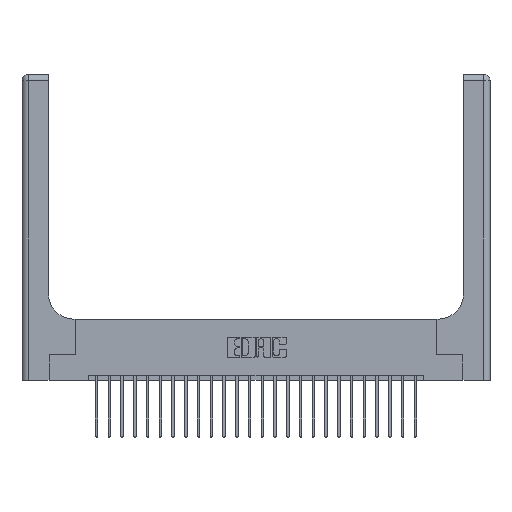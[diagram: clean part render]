
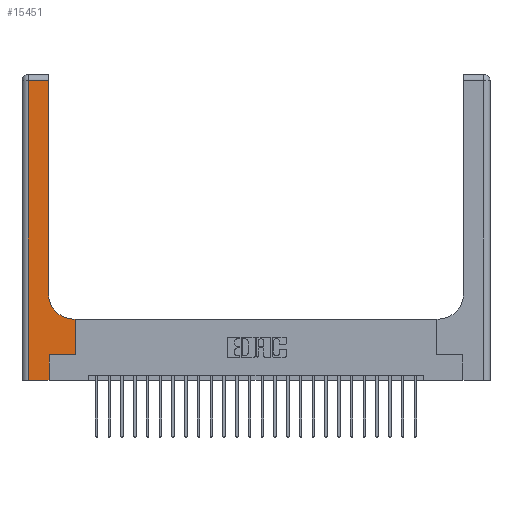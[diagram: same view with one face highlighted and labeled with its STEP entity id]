
A CAD part, top view. The second image highlights one B-rep face of the part: STEP entity #15451.
In plain terms, the highlighted planar face has unit normal (0, 0, 1).
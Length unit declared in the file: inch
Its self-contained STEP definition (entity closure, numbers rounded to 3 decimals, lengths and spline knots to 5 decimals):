
#1 = LINE ( 'NONE', #17012, #22369 ) ;
#165 = CARTESIAN_POINT ( 'NONE',  ( 0.26, 2.94, 0.37 ) ) ;
#623 = CARTESIAN_POINT ( 'NONE',  ( 0.06, 0., 0.37 ) ) ;
#660 = VECTOR ( 'NONE', #21914, 39.37008 ) ;
#692 = ORIENTED_EDGE ( 'NONE', *, *, #14863, .T. ) ;
#721 = DIRECTION ( 'NONE',  ( 0., 1., 0. ) ) ;
#759 = VECTOR ( 'NONE', #11160, 39.37008 ) ;
#1568 = DIRECTION ( 'NONE',  ( 0., 0., -1. ) ) ;
#1949 = DIRECTION ( 'NONE',  ( -1., 0., 0. ) ) ;
#2361 = DIRECTION ( 'NONE',  ( 0., 1., 0. ) ) ;
#2493 = VERTEX_POINT ( 'NONE', #22135 ) ;
#2516 = LINE ( 'NONE', #21000, #11321 ) ;
#2921 = EDGE_LOOP ( 'NONE', ( #4678, #18273, #2970, #3526, #19930, #16629, #23258, #692, #19348 ) ) ;
#2970 = ORIENTED_EDGE ( 'NONE', *, *, #20017, .T. ) ;
#2985 = EDGE_CURVE ( 'NONE', #14610, #8195, #4981, .T. ) ;
#3526 = ORIENTED_EDGE ( 'NONE', *, *, #21913, .T. ) ;
#4008 = DIRECTION ( 'NONE',  ( 0., -1., 0. ) ) ;
#4084 = CARTESIAN_POINT ( 'NONE',  ( 0.06, 3., 0.37 ) ) ;
#4603 = LINE ( 'NONE', #13674, #11667 ) ;
#4678 = ORIENTED_EDGE ( 'NONE', *, *, #7234, .T. ) ;
#4731 = VERTEX_POINT ( 'NONE', #165 ) ;
#4958 = VERTEX_POINT ( 'NONE', #623 ) ;
#4981 = LINE ( 'NONE', #6660, #18753 ) ;
#5640 = CARTESIAN_POINT ( 'NONE',  ( 0., 3., 0.37 ) ) ;
#5770 = LINE ( 'NONE', #13314, #759 ) ;
#5852 = EDGE_CURVE ( 'NONE', #23326, #8071, #8689, .T. ) ;
#6180 = CARTESIAN_POINT ( 'NONE',  ( 0.26, 3., 0.37 ) ) ;
#6660 = CARTESIAN_POINT ( 'NONE',  ( 0.528, 0.25, 0.37 ) ) ;
#6715 = CARTESIAN_POINT ( 'NONE',  ( 0.26, 0.85, 0.37 ) ) ;
#7234 = EDGE_CURVE ( 'NONE', #8071, #4731, #16229, .T. ) ;
#8071 = VERTEX_POINT ( 'NONE', #6715 ) ;
#8195 = VERTEX_POINT ( 'NONE', #9069 ) ;
#8203 = VECTOR ( 'NONE', #4008, 39.37008 ) ;
#8394 = FACE_OUTER_BOUND ( 'NONE', #2921, .T. ) ;
#8689 = CIRCLE ( 'NONE', #9974, 0.25 ) ;
#8897 = CARTESIAN_POINT ( 'NONE',  ( 0.51, 0.85, 0.37 ) ) ;
#9069 = CARTESIAN_POINT ( 'NONE',  ( 0.528, 0.6, 0.37 ) ) ;
#9901 = CARTESIAN_POINT ( 'NONE',  ( 0.51, 0.6, 0.37 ) ) ;
#9974 = AXIS2_PLACEMENT_3D ( 'NONE', #8897, #1568, #22182 ) ;
#10368 = LINE ( 'NONE', #10765, #660 ) ;
#10765 = CARTESIAN_POINT ( 'NONE',  ( 0., 0., 0.37 ) ) ;
#11034 = VERTEX_POINT ( 'NONE', #14365 ) ;
#11160 = DIRECTION ( 'NONE',  ( 1., 0., 0. ) ) ;
#11248 = CARTESIAN_POINT ( 'NONE',  ( 0.528, 0.25, 0.37 ) ) ;
#11321 = VECTOR ( 'NONE', #19107, 39.37008 ) ;
#11667 = VECTOR ( 'NONE', #2361, 39.37008 ) ;
#13248 = AXIS2_PLACEMENT_3D ( 'NONE', #5640, #13293, #1949 ) ;
#13293 = DIRECTION ( 'NONE',  ( 0., 0., -1. ) ) ;
#13314 = CARTESIAN_POINT ( 'NONE',  ( 0.265, 0.25, 0.37 ) ) ;
#13674 = CARTESIAN_POINT ( 'NONE',  ( 0.265, 0., 0.37 ) ) ;
#14365 = CARTESIAN_POINT ( 'NONE',  ( 0.06, 2.94, 0.37 ) ) ;
#14424 = EDGE_CURVE ( 'NONE', #20872, #2493, #4603, .T. ) ;
#14563 = EDGE_CURVE ( 'NONE', #2493, #14610, #5770, .T. ) ;
#14610 = VERTEX_POINT ( 'NONE', #11248 ) ;
#14863 = EDGE_CURVE ( 'NONE', #8195, #23326, #2516, .T. ) ;
#15451 = ADVANCED_FACE ( 'NONE', ( #8394 ), #22705, .F. ) ;
#15654 = VECTOR ( 'NONE', #19519, 39.37008 ) ;
#16229 = LINE ( 'NONE', #6180, #15654 ) ;
#16629 = ORIENTED_EDGE ( 'NONE', *, *, #14563, .T. ) ;
#17012 = CARTESIAN_POINT ( 'NONE',  ( 0., 2.94, 0.37 ) ) ;
#18273 = ORIENTED_EDGE ( 'NONE', *, *, #22746, .T. ) ;
#18753 = VECTOR ( 'NONE', #721, 39.37008 ) ;
#19107 = DIRECTION ( 'NONE',  ( -1., 0., 0. ) ) ;
#19348 = ORIENTED_EDGE ( 'NONE', *, *, #5852, .T. ) ;
#19519 = DIRECTION ( 'NONE',  ( 0., 1., 0. ) ) ;
#19930 = ORIENTED_EDGE ( 'NONE', *, *, #14424, .T. ) ;
#20017 = EDGE_CURVE ( 'NONE', #11034, #4958, #20797, .T. ) ;
#20641 = DIRECTION ( 'NONE',  ( -1., 0., 0. ) ) ;
#20797 = LINE ( 'NONE', #4084, #8203 ) ;
#20872 = VERTEX_POINT ( 'NONE', #20895 ) ;
#20895 = CARTESIAN_POINT ( 'NONE',  ( 0.265, 0., 0.37 ) ) ;
#21000 = CARTESIAN_POINT ( 'NONE',  ( 0.26, 0.6, 0.37 ) ) ;
#21913 = EDGE_CURVE ( 'NONE', #4958, #20872, #10368, .T. ) ;
#21914 = DIRECTION ( 'NONE',  ( 1., 0., 0. ) ) ;
#22135 = CARTESIAN_POINT ( 'NONE',  ( 0.265, 0.25, 0.37 ) ) ;
#22182 = DIRECTION ( 'NONE',  ( 1., 0., 0. ) ) ;
#22369 = VECTOR ( 'NONE', #20641, 39.37008 ) ;
#22705 = PLANE ( 'NONE',  #13248 ) ;
#22746 = EDGE_CURVE ( 'NONE', #4731, #11034, #1, .T. ) ;
#23258 = ORIENTED_EDGE ( 'NONE', *, *, #2985, .T. ) ;
#23326 = VERTEX_POINT ( 'NONE', #9901 ) ;
